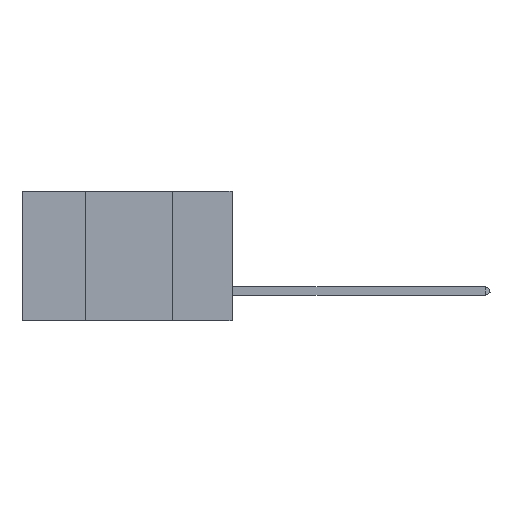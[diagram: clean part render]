
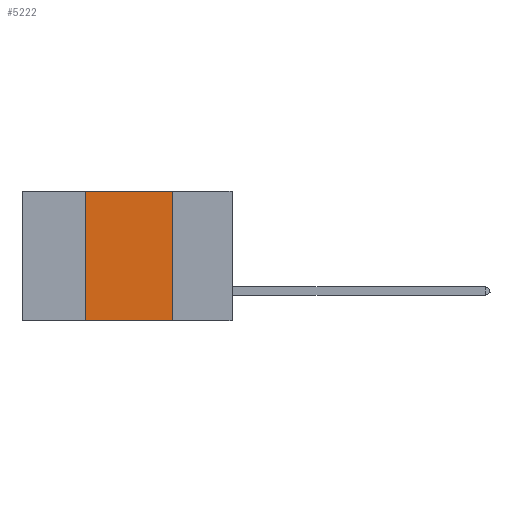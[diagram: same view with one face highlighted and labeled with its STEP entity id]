
A CAD part, left-side view. The second image highlights one B-rep face of the part: STEP entity #5222.
In plain terms, the highlighted planar face has unit normal (-1, 0, 0).
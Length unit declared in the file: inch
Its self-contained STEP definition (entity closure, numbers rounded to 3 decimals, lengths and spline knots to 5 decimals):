
#621 = EDGE_CURVE ( 'NONE', #12909, #3996, #2067, .T. ) ;
#1236 = LINE ( 'NONE', #10246, #11572 ) ;
#1669 = DIRECTION ( 'NONE',  ( 0., 0., -1. ) ) ;
#2067 = LINE ( 'NONE', #24667, #15938 ) ;
#3996 = VERTEX_POINT ( 'NONE', #24716 ) ;
#4514 = ORIENTED_EDGE ( 'NONE', *, *, #24790, .F. ) ;
#4572 = EDGE_CURVE ( 'NONE', #5190, #3996, #22590, .T. ) ;
#5190 = VERTEX_POINT ( 'NONE', #5641 ) ;
#5222 = ADVANCED_FACE ( 'NONE', ( #21922 ), #19820, .F. ) ;
#5609 = AXIS2_PLACEMENT_3D ( 'NONE', #7680, #24103, #26065 ) ;
#5641 = CARTESIAN_POINT ( 'NONE',  ( 0., 0.17, 0. ) ) ;
#5727 = CARTESIAN_POINT ( 'NONE',  ( 0., 0.17, 0. ) ) ;
#6816 = LINE ( 'NONE', #16414, #8428 ) ;
#7680 = CARTESIAN_POINT ( 'NONE',  ( 0., 0.6, 0. ) ) ;
#7946 = ORIENTED_EDGE ( 'NONE', *, *, #621, .T. ) ;
#8089 = DIRECTION ( 'NONE',  ( 0., -1., 0. ) ) ;
#8428 = VECTOR ( 'NONE', #16061, 39.37008 ) ;
#10246 = CARTESIAN_POINT ( 'NONE',  ( 0., 0.6, 0. ) ) ;
#10626 = EDGE_CURVE ( 'NONE', #12909, #16739, #6816, .T. ) ;
#11572 = VECTOR ( 'NONE', #8089, 39.37008 ) ;
#12228 = CARTESIAN_POINT ( 'NONE',  ( 0., 0.42, 0. ) ) ;
#12909 = VERTEX_POINT ( 'NONE', #24775 ) ;
#15795 = EDGE_LOOP ( 'NONE', ( #16319, #4514, #21565, #7946 ) ) ;
#15938 = VECTOR ( 'NONE', #22633, 39.37008 ) ;
#16061 = DIRECTION ( 'NONE',  ( 0., 0., 1. ) ) ;
#16319 = ORIENTED_EDGE ( 'NONE', *, *, #4572, .F. ) ;
#16414 = CARTESIAN_POINT ( 'NONE',  ( 0., 0.42, 0. ) ) ;
#16739 = VERTEX_POINT ( 'NONE', #12228 ) ;
#18050 = VECTOR ( 'NONE', #1669, 39.37008 ) ;
#19820 = PLANE ( 'NONE',  #5609 ) ;
#21565 = ORIENTED_EDGE ( 'NONE', *, *, #10626, .F. ) ;
#21922 = FACE_OUTER_BOUND ( 'NONE', #15795, .T. ) ;
#22590 = LINE ( 'NONE', #5727, #18050 ) ;
#22633 = DIRECTION ( 'NONE',  ( 0., -1., 0. ) ) ;
#24103 = DIRECTION ( 'NONE',  ( 1., 0., 0. ) ) ;
#24667 = CARTESIAN_POINT ( 'NONE',  ( 0., 0.6, -0.37 ) ) ;
#24716 = CARTESIAN_POINT ( 'NONE',  ( 0., 0.17, -0.37 ) ) ;
#24775 = CARTESIAN_POINT ( 'NONE',  ( 0., 0.42, -0.37 ) ) ;
#24790 = EDGE_CURVE ( 'NONE', #16739, #5190, #1236, .T. ) ;
#26065 = DIRECTION ( 'NONE',  ( 0., 0., -1. ) ) ;
